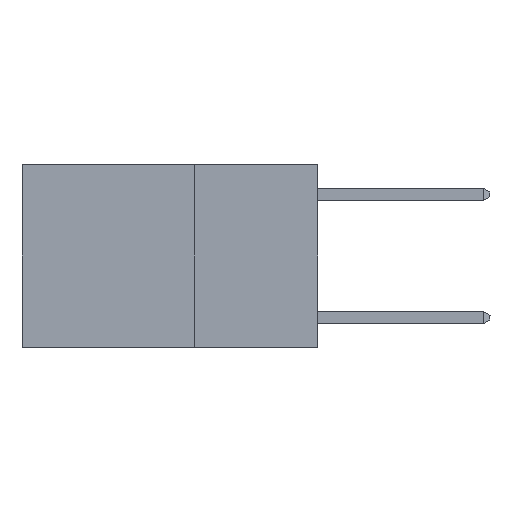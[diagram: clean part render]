
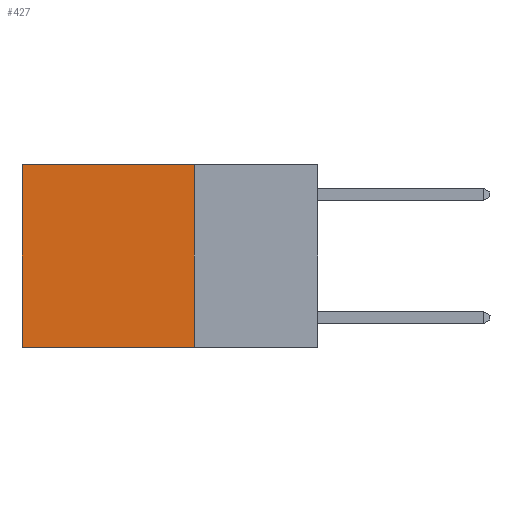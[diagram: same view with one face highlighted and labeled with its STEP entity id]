
A CAD part, left-side view. The second image highlights one B-rep face of the part: STEP entity #427.
In plain terms, the highlighted planar face has unit normal (-1, 0, 0).
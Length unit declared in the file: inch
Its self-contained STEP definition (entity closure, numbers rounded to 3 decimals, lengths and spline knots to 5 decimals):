
#410 = AXIS2_PLACEMENT_3D ( 'NONE', #5022, #5350, #9907 ) ;
#416 = LINE ( 'NONE', #2549, #8583 ) ;
#427 = ADVANCED_FACE ( 'NONE', ( #2701 ), #9768, .F. ) ;
#870 = ORIENTED_EDGE ( 'NONE', *, *, #4387, .F. ) ;
#943 = DIRECTION ( 'NONE',  ( 0., 0., -1. ) ) ;
#1064 = VECTOR ( 'NONE', #5055, 39.37008 ) ;
#1813 = ORIENTED_EDGE ( 'NONE', *, *, #9087, .T. ) ;
#2426 = LINE ( 'NONE', #2893, #8201 ) ;
#2549 = CARTESIAN_POINT ( 'NONE',  ( 0.2625, 0.25, 0. ) ) ;
#2607 = CARTESIAN_POINT ( 'NONE',  ( 0.2625, 0.6, 0. ) ) ;
#2701 = FACE_OUTER_BOUND ( 'NONE', #6201, .T. ) ;
#2789 = EDGE_CURVE ( 'NONE', #6879, #5198, #3533, .T. ) ;
#2893 = CARTESIAN_POINT ( 'NONE',  ( 0.2625, 0.25, 0. ) ) ;
#2995 = CARTESIAN_POINT ( 'NONE',  ( 0.2625, 0.25, 0. ) ) ;
#3533 = LINE ( 'NONE', #5807, #1064 ) ;
#3833 = VERTEX_POINT ( 'NONE', #6621 ) ;
#4387 = EDGE_CURVE ( 'NONE', #4582, #6879, #416, .T. ) ;
#4582 = VERTEX_POINT ( 'NONE', #2995 ) ;
#5022 = CARTESIAN_POINT ( 'NONE',  ( 0.2625, 0.25, 0. ) ) ;
#5055 = DIRECTION ( 'NONE',  ( 0., 1., 0. ) ) ;
#5198 = VERTEX_POINT ( 'NONE', #9965 ) ;
#5300 = VECTOR ( 'NONE', #943, 39.37008 ) ;
#5350 = DIRECTION ( 'NONE',  ( 1., 0., 0. ) ) ;
#5807 = CARTESIAN_POINT ( 'NONE',  ( 0.2625, 0.25, -0.37 ) ) ;
#6068 = ORIENTED_EDGE ( 'NONE', *, *, #2789, .F. ) ;
#6201 = EDGE_LOOP ( 'NONE', ( #7788, #6068, #870, #1813 ) ) ;
#6621 = CARTESIAN_POINT ( 'NONE',  ( 0.2625, 0.6, 0. ) ) ;
#6879 = VERTEX_POINT ( 'NONE', #8486 ) ;
#7274 = LINE ( 'NONE', #2607, #5300 ) ;
#7362 = EDGE_CURVE ( 'NONE', #3833, #5198, #7274, .T. ) ;
#7525 = DIRECTION ( 'NONE',  ( 0., 0., -1. ) ) ;
#7788 = ORIENTED_EDGE ( 'NONE', *, *, #7362, .T. ) ;
#8201 = VECTOR ( 'NONE', #8342, 39.37008 ) ;
#8342 = DIRECTION ( 'NONE',  ( 0., 1., 0. ) ) ;
#8486 = CARTESIAN_POINT ( 'NONE',  ( 0.2625, 0.25, -0.37 ) ) ;
#8583 = VECTOR ( 'NONE', #7525, 39.37008 ) ;
#9087 = EDGE_CURVE ( 'NONE', #4582, #3833, #2426, .T. ) ;
#9768 = PLANE ( 'NONE',  #410 ) ;
#9907 = DIRECTION ( 'NONE',  ( 0., 0., -1. ) ) ;
#9965 = CARTESIAN_POINT ( 'NONE',  ( 0.2625, 0.6, -0.37 ) ) ;
